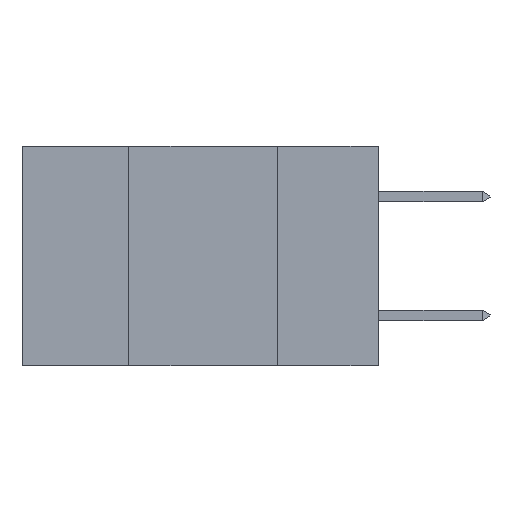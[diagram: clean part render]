
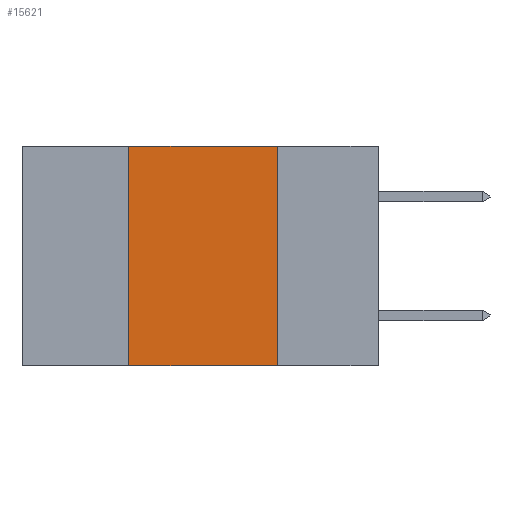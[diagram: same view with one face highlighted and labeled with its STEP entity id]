
A CAD part, left-side view. The second image highlights one B-rep face of the part: STEP entity #15621.
In plain terms, the highlighted planar face has unit normal (-1, 0, 0).
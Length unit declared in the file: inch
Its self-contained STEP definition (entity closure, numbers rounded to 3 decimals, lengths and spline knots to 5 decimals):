
#298 = AXIS2_PLACEMENT_3D ( 'NONE', #29623, #17572, #24813 ) ;
#877 = VERTEX_POINT ( 'NONE', #9221 ) ;
#879 = EDGE_CURVE ( 'NONE', #22924, #877, #18225, .T. ) ;
#1151 = EDGE_LOOP ( 'NONE', ( #26849, #7788, #9355, #21247 ) ) ;
#1363 = CARTESIAN_POINT ( 'NONE',  ( 0., 0.17, -0.37 ) ) ;
#2673 = VERTEX_POINT ( 'NONE', #6253 ) ;
#2938 = LINE ( 'NONE', #14449, #4386 ) ;
#2951 = DIRECTION ( 'NONE',  ( 0., 0., -1. ) ) ;
#4386 = VECTOR ( 'NONE', #2951, 39.37008 ) ;
#4548 = VERTEX_POINT ( 'NONE', #1363 ) ;
#5718 = VECTOR ( 'NONE', #16298, 39.37008 ) ;
#6253 = CARTESIAN_POINT ( 'NONE',  ( 0., 0.17, 0. ) ) ;
#7788 = ORIENTED_EDGE ( 'NONE', *, *, #29215, .F. ) ;
#9000 = CARTESIAN_POINT ( 'NONE',  ( 0., 0.6, 0. ) ) ;
#9221 = CARTESIAN_POINT ( 'NONE',  ( 0., 0.42, 0. ) ) ;
#9355 = ORIENTED_EDGE ( 'NONE', *, *, #879, .F. ) ;
#10058 = CARTESIAN_POINT ( 'NONE',  ( 0., 0.6, -0.37 ) ) ;
#10276 = LINE ( 'NONE', #9000, #21327 ) ;
#14449 = CARTESIAN_POINT ( 'NONE',  ( 0., 0.17, 0. ) ) ;
#15621 = ADVANCED_FACE ( 'NONE', ( #21013 ), #17758, .F. ) ;
#16298 = DIRECTION ( 'NONE',  ( 0., 0., 1. ) ) ;
#17572 = DIRECTION ( 'NONE',  ( 1., 0., 0. ) ) ;
#17758 = PLANE ( 'NONE',  #298 ) ;
#18225 = LINE ( 'NONE', #27930, #5718 ) ;
#18767 = EDGE_CURVE ( 'NONE', #22924, #4548, #21910, .T. ) ;
#20799 = VECTOR ( 'NONE', #26263, 39.37008 ) ;
#21013 = FACE_OUTER_BOUND ( 'NONE', #1151, .T. ) ;
#21247 = ORIENTED_EDGE ( 'NONE', *, *, #18767, .T. ) ;
#21327 = VECTOR ( 'NONE', #27411, 39.37008 ) ;
#21910 = LINE ( 'NONE', #10058, #20799 ) ;
#22924 = VERTEX_POINT ( 'NONE', #25422 ) ;
#24147 = EDGE_CURVE ( 'NONE', #2673, #4548, #2938, .T. ) ;
#24813 = DIRECTION ( 'NONE',  ( 0., 0., -1. ) ) ;
#25422 = CARTESIAN_POINT ( 'NONE',  ( 0., 0.42, -0.37 ) ) ;
#26263 = DIRECTION ( 'NONE',  ( 0., -1., 0. ) ) ;
#26849 = ORIENTED_EDGE ( 'NONE', *, *, #24147, .F. ) ;
#27411 = DIRECTION ( 'NONE',  ( 0., -1., 0. ) ) ;
#27930 = CARTESIAN_POINT ( 'NONE',  ( 0., 0.42, 0. ) ) ;
#29215 = EDGE_CURVE ( 'NONE', #877, #2673, #10276, .T. ) ;
#29623 = CARTESIAN_POINT ( 'NONE',  ( 0., 0.6, 0. ) ) ;
